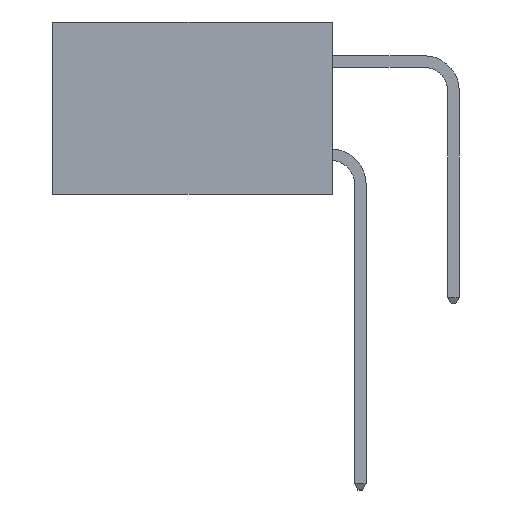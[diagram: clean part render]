
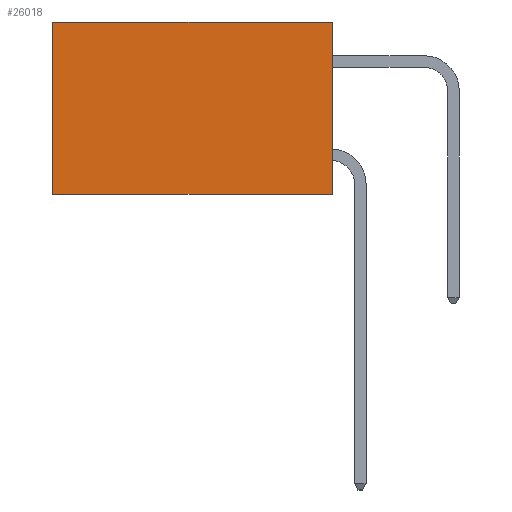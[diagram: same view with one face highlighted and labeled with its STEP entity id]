
A CAD part, left-side view. The second image highlights one B-rep face of the part: STEP entity #26018.
In plain terms, the highlighted planar face has unit normal (-1, 0, 0).
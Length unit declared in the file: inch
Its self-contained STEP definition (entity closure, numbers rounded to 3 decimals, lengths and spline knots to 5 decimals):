
#2930 = VERTEX_POINT ( 'NONE', #9889 ) ;
#3002 = EDGE_CURVE ( 'NONE', #7342, #16264, #8689, .T. ) ;
#4207 = LINE ( 'NONE', #6920, #25522 ) ;
#4437 = AXIS2_PLACEMENT_3D ( 'NONE', #11545, #26087, #13725 ) ;
#5275 = LINE ( 'NONE', #7167, #10136 ) ;
#6105 = CARTESIAN_POINT ( 'NONE',  ( 0.2615, 0.6, -0.37 ) ) ;
#6920 = CARTESIAN_POINT ( 'NONE',  ( 0.2615, 0., -0.37 ) ) ;
#7167 = CARTESIAN_POINT ( 'NONE',  ( 0.2615, 0., 0. ) ) ;
#7342 = VERTEX_POINT ( 'NONE', #9371 ) ;
#7903 = EDGE_LOOP ( 'NONE', ( #15780, #21593, #13350, #11022 ) ) ;
#8115 = LINE ( 'NONE', #8770, #17814 ) ;
#8689 = LINE ( 'NONE', #6105, #13554 ) ;
#8770 = CARTESIAN_POINT ( 'NONE',  ( 0.2615, 0., -0.37 ) ) ;
#9259 = DIRECTION ( 'NONE',  ( 0., 1., 0. ) ) ;
#9371 = CARTESIAN_POINT ( 'NONE',  ( 0.2615, 0.6, 0. ) ) ;
#9889 = CARTESIAN_POINT ( 'NONE',  ( 0.2615, 0., -0.37 ) ) ;
#10136 = VECTOR ( 'NONE', #9259, 39.37008 ) ;
#11022 = ORIENTED_EDGE ( 'NONE', *, *, #24764, .T. ) ;
#11172 = DIRECTION ( 'NONE',  ( 0., 1., 0. ) ) ;
#11545 = CARTESIAN_POINT ( 'NONE',  ( 0.2615, 0., -0.37 ) ) ;
#11639 = PLANE ( 'NONE',  #4437 ) ;
#13312 = CARTESIAN_POINT ( 'NONE',  ( 0.2615, 0., 0. ) ) ;
#13350 = ORIENTED_EDGE ( 'NONE', *, *, #17571, .F. ) ;
#13554 = VECTOR ( 'NONE', #18480, 39.37008 ) ;
#13725 = DIRECTION ( 'NONE',  ( 0., 0., -1. ) ) ;
#15780 = ORIENTED_EDGE ( 'NONE', *, *, #3002, .T. ) ;
#16264 = VERTEX_POINT ( 'NONE', #18503 ) ;
#17103 = VERTEX_POINT ( 'NONE', #13312 ) ;
#17571 = EDGE_CURVE ( 'NONE', #17103, #2930, #8115, .T. ) ;
#17814 = VECTOR ( 'NONE', #21135, 39.37008 ) ;
#18480 = DIRECTION ( 'NONE',  ( 0., 0., -1. ) ) ;
#18503 = CARTESIAN_POINT ( 'NONE',  ( 0.2615, 0.6, -0.37 ) ) ;
#21135 = DIRECTION ( 'NONE',  ( 0., 0., -1. ) ) ;
#21593 = ORIENTED_EDGE ( 'NONE', *, *, #26616, .F. ) ;
#24764 = EDGE_CURVE ( 'NONE', #17103, #7342, #5275, .T. ) ;
#25522 = VECTOR ( 'NONE', #11172, 39.37008 ) ;
#25887 = FACE_OUTER_BOUND ( 'NONE', #7903, .T. ) ;
#26018 = ADVANCED_FACE ( 'NONE', ( #25887 ), #11639, .F. ) ;
#26087 = DIRECTION ( 'NONE',  ( 1., 0., 0. ) ) ;
#26616 = EDGE_CURVE ( 'NONE', #2930, #16264, #4207, .T. ) ;
